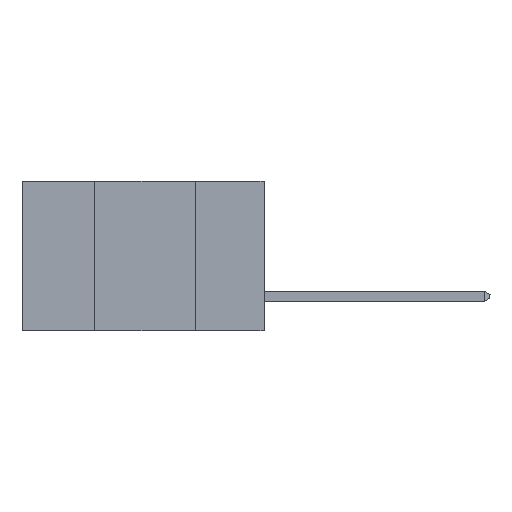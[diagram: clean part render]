
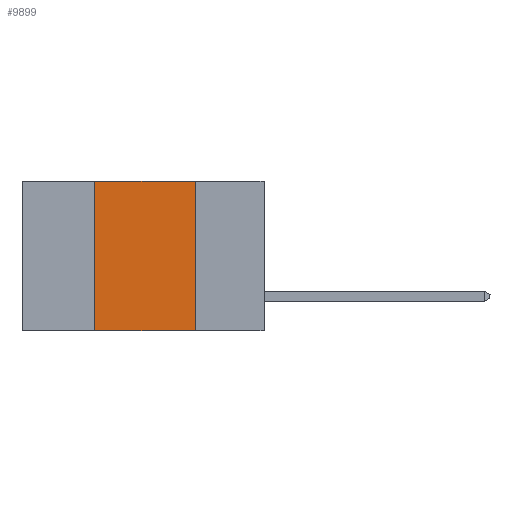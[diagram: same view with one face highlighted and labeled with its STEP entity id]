
A CAD part, left-side view. The second image highlights one B-rep face of the part: STEP entity #9899.
In plain terms, the highlighted planar face has unit normal (-1, 0, 0).
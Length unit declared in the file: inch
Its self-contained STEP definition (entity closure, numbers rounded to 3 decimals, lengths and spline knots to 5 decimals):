
#151 = VERTEX_POINT ( 'NONE', #13612 ) ;
#165 = DIRECTION ( 'NONE',  ( 0., 0., -1. ) ) ;
#764 = VECTOR ( 'NONE', #165, 39.37008 ) ;
#1053 = VECTOR ( 'NONE', #9870, 39.37008 ) ;
#1382 = LINE ( 'NONE', #4935, #1053 ) ;
#1595 = VECTOR ( 'NONE', #9804, 39.37008 ) ;
#2073 = CARTESIAN_POINT ( 'NONE',  ( 0., 0.42, -0.37 ) ) ;
#2458 = VERTEX_POINT ( 'NONE', #6886 ) ;
#2659 = VECTOR ( 'NONE', #2985, 39.37008 ) ;
#2985 = DIRECTION ( 'NONE',  ( 0., 0., 1. ) ) ;
#3150 = ORIENTED_EDGE ( 'NONE', *, *, #11297, .F. ) ;
#3829 = CARTESIAN_POINT ( 'NONE',  ( 0., 0.6, 0. ) ) ;
#4575 = VERTEX_POINT ( 'NONE', #4757 ) ;
#4706 = DIRECTION ( 'NONE',  ( 1., 0., 0. ) ) ;
#4757 = CARTESIAN_POINT ( 'NONE',  ( 0., 0.17, -0.37 ) ) ;
#4935 = CARTESIAN_POINT ( 'NONE',  ( 0., 0.6, -0.37 ) ) ;
#5100 = CARTESIAN_POINT ( 'NONE',  ( 0., 0.6, 0. ) ) ;
#5918 = EDGE_LOOP ( 'NONE', ( #7309, #3150, #14514, #6785 ) ) ;
#6785 = ORIENTED_EDGE ( 'NONE', *, *, #9947, .T. ) ;
#6886 = CARTESIAN_POINT ( 'NONE',  ( 0., 0.42, 0. ) ) ;
#7309 = ORIENTED_EDGE ( 'NONE', *, *, #15015, .F. ) ;
#9394 = VERTEX_POINT ( 'NONE', #2073 ) ;
#9804 = DIRECTION ( 'NONE',  ( 0., -1., 0. ) ) ;
#9870 = DIRECTION ( 'NONE',  ( 0., -1., 0. ) ) ;
#9899 = ADVANCED_FACE ( 'NONE', ( #10435 ), #14110, .F. ) ;
#9947 = EDGE_CURVE ( 'NONE', #9394, #4575, #1382, .T. ) ;
#10435 = FACE_OUTER_BOUND ( 'NONE', #5918, .T. ) ;
#10710 = LINE ( 'NONE', #10944, #764 ) ;
#10944 = CARTESIAN_POINT ( 'NONE',  ( 0., 0.17, -0.37 ) ) ;
#11055 = DIRECTION ( 'NONE',  ( 0., 0., -1. ) ) ;
#11297 = EDGE_CURVE ( 'NONE', #2458, #151, #13452, .T. ) ;
#11951 = AXIS2_PLACEMENT_3D ( 'NONE', #3829, #4706, #11055 ) ;
#12758 = LINE ( 'NONE', #14927, #2659 ) ;
#13452 = LINE ( 'NONE', #5100, #1595 ) ;
#13612 = CARTESIAN_POINT ( 'NONE',  ( 0., 0.17, 0. ) ) ;
#14001 = EDGE_CURVE ( 'NONE', #9394, #2458, #12758, .T. ) ;
#14110 = PLANE ( 'NONE',  #11951 ) ;
#14514 = ORIENTED_EDGE ( 'NONE', *, *, #14001, .F. ) ;
#14927 = CARTESIAN_POINT ( 'NONE',  ( 0., 0.42, -0.37 ) ) ;
#15015 = EDGE_CURVE ( 'NONE', #151, #4575, #10710, .T. ) ;
